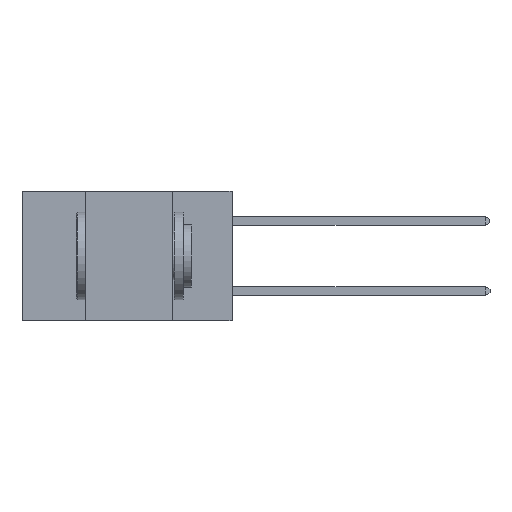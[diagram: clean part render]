
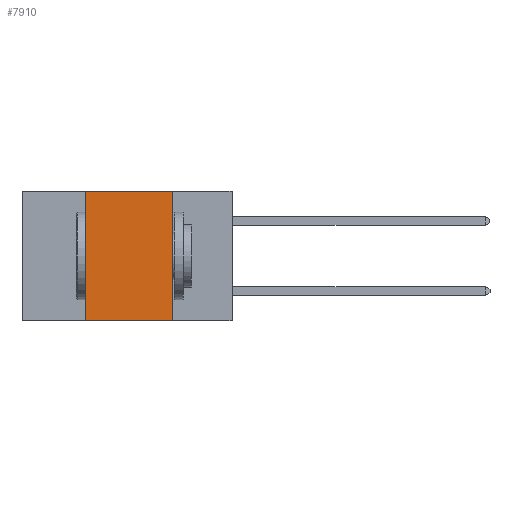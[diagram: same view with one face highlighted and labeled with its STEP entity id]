
A CAD part, left-side view. The second image highlights one B-rep face of the part: STEP entity #7910.
In plain terms, the highlighted planar face has unit normal (-1, 0, 0).
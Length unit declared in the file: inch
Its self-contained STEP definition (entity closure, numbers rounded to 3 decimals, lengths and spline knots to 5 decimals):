
#122 = ORIENTED_EDGE ( 'NONE', *, *, #7031, .T. ) ;
#1044 = DIRECTION ( 'NONE',  ( 0., -1., 0. ) ) ;
#1460 = CARTESIAN_POINT ( 'NONE',  ( 0., 0.6, -0.37 ) ) ;
#1967 = CARTESIAN_POINT ( 'NONE',  ( 0., 0.42, 0. ) ) ;
#2104 = LINE ( 'NONE', #2710, #4390 ) ;
#2194 = DIRECTION ( 'NONE',  ( 1., 0., 0. ) ) ;
#2393 = EDGE_CURVE ( 'NONE', #7782, #13292, #2104, .T. ) ;
#2610 = DIRECTION ( 'NONE',  ( 0., 0., -1. ) ) ;
#2710 = CARTESIAN_POINT ( 'NONE',  ( 0., 0.17, 0. ) ) ;
#3506 = DIRECTION ( 'NONE',  ( 0., -1., 0. ) ) ;
#3640 = CARTESIAN_POINT ( 'NONE',  ( 0., 0.6, 0. ) ) ;
#4390 = VECTOR ( 'NONE', #2610, 39.37008 ) ;
#4434 = ORIENTED_EDGE ( 'NONE', *, *, #2393, .F. ) ;
#4839 = CARTESIAN_POINT ( 'NONE',  ( 0., 0.42, 0. ) ) ;
#4984 = DIRECTION ( 'NONE',  ( 0., 0., 1. ) ) ;
#5794 = ORIENTED_EDGE ( 'NONE', *, *, #6343, .F. ) ;
#6343 = EDGE_CURVE ( 'NONE', #10948, #12504, #10183, .T. ) ;
#6418 = EDGE_CURVE ( 'NONE', #12504, #7782, #7467, .T. ) ;
#6686 = AXIS2_PLACEMENT_3D ( 'NONE', #13327, #2194, #9583 ) ;
#6957 = CARTESIAN_POINT ( 'NONE',  ( 0., 0.17, -0.37 ) ) ;
#7031 = EDGE_CURVE ( 'NONE', #10948, #13292, #12706, .T. ) ;
#7134 = VECTOR ( 'NONE', #3506, 39.37008 ) ;
#7467 = LINE ( 'NONE', #3640, #7134 ) ;
#7782 = VERTEX_POINT ( 'NONE', #9367 ) ;
#7910 = ADVANCED_FACE ( 'NONE', ( #10884 ), #8614, .F. ) ;
#8226 = EDGE_LOOP ( 'NONE', ( #4434, #10465, #5794, #122 ) ) ;
#8614 = PLANE ( 'NONE',  #6686 ) ;
#9367 = CARTESIAN_POINT ( 'NONE',  ( 0., 0.17, 0. ) ) ;
#9583 = DIRECTION ( 'NONE',  ( 0., 0., -1. ) ) ;
#10183 = LINE ( 'NONE', #4839, #12702 ) ;
#10186 = VECTOR ( 'NONE', #1044, 39.37008 ) ;
#10465 = ORIENTED_EDGE ( 'NONE', *, *, #6418, .F. ) ;
#10884 = FACE_OUTER_BOUND ( 'NONE', #8226, .T. ) ;
#10948 = VERTEX_POINT ( 'NONE', #12736 ) ;
#12504 = VERTEX_POINT ( 'NONE', #1967 ) ;
#12702 = VECTOR ( 'NONE', #4984, 39.37008 ) ;
#12706 = LINE ( 'NONE', #1460, #10186 ) ;
#12736 = CARTESIAN_POINT ( 'NONE',  ( 0., 0.42, -0.37 ) ) ;
#13292 = VERTEX_POINT ( 'NONE', #6957 ) ;
#13327 = CARTESIAN_POINT ( 'NONE',  ( 0., 0.6, 0. ) ) ;
